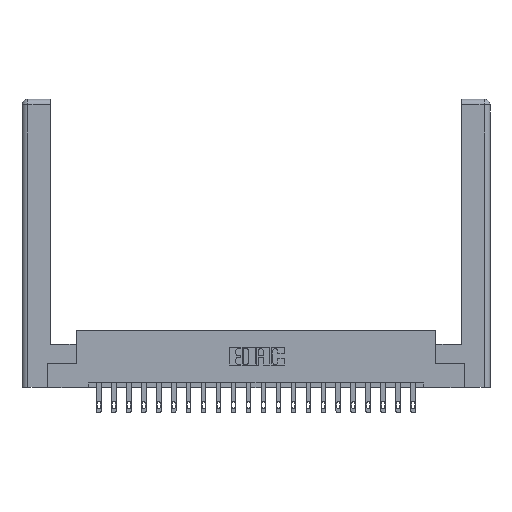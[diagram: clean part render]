
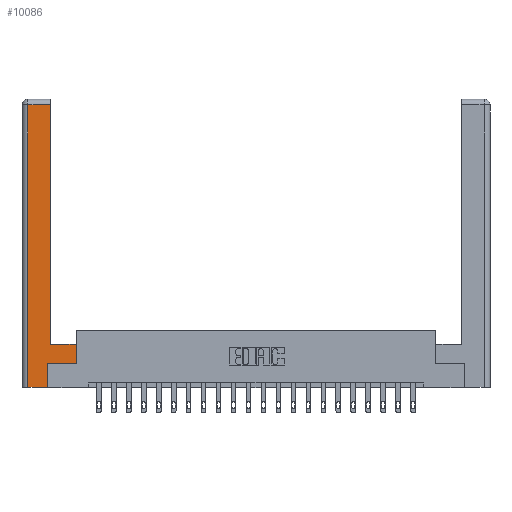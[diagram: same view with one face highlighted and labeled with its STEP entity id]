
A CAD part, top view. The second image highlights one B-rep face of the part: STEP entity #10086.
In plain terms, the highlighted planar face has unit normal (0, 0, 1).
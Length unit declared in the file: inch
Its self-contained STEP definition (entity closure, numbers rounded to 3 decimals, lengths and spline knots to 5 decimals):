
#191 = CARTESIAN_POINT ( 'NONE',  ( 0.565, 0.45, 0. ) ) ;
#448 = CARTESIAN_POINT ( 'NONE',  ( 0.295, 2.94, 0. ) ) ;
#465 = ORIENTED_EDGE ( 'NONE', *, *, #10712, .T. ) ;
#911 = LINE ( 'NONE', #21684, #7870 ) ;
#932 = ORIENTED_EDGE ( 'NONE', *, *, #4241, .T. ) ;
#980 = DIRECTION ( 'NONE',  ( 1., 0., 0. ) ) ;
#1109 = CARTESIAN_POINT ( 'NONE',  ( 0.0615, 2.94, 0. ) ) ;
#1125 = VERTEX_POINT ( 'NONE', #8015 ) ;
#2130 = CARTESIAN_POINT ( 'NONE',  ( 0.295, 0.45, 0. ) ) ;
#2288 = DIRECTION ( 'NONE',  ( -1., 0., 0. ) ) ;
#2538 = ORIENTED_EDGE ( 'NONE', *, *, #7985, .T. ) ;
#2621 = CARTESIAN_POINT ( 'NONE',  ( 0.565, 0.245, 0. ) ) ;
#3746 = VECTOR ( 'NONE', #13568, 39.37008 ) ;
#3827 = CARTESIAN_POINT ( 'NONE',  ( 0.295, 0.45, 0. ) ) ;
#4241 = EDGE_CURVE ( 'NONE', #12772, #1125, #19651, .T. ) ;
#4307 = EDGE_CURVE ( 'NONE', #20152, #16746, #19106, .T. ) ;
#4460 = DIRECTION ( 'NONE',  ( 0., 1., 0. ) ) ;
#4882 = DIRECTION ( 'NONE',  ( 0., -1., 0. ) ) ;
#5393 = VERTEX_POINT ( 'NONE', #7717 ) ;
#5570 = VECTOR ( 'NONE', #4882, 39.37008 ) ;
#6039 = CARTESIAN_POINT ( 'NONE',  ( 0.295, 3., 0. ) ) ;
#6132 = VECTOR ( 'NONE', #18118, 39.37008 ) ;
#6520 = ORIENTED_EDGE ( 'NONE', *, *, #15748, .T. ) ;
#6770 = ORIENTED_EDGE ( 'NONE', *, *, #7977, .T. ) ;
#7197 = LINE ( 'NONE', #9869, #5570 ) ;
#7478 = CARTESIAN_POINT ( 'NONE',  ( 0.0615, 2.94, 0. ) ) ;
#7717 = CARTESIAN_POINT ( 'NONE',  ( 0.565, 0.45, 0. ) ) ;
#7759 = DIRECTION ( 'NONE',  ( -1., 0., 0. ) ) ;
#7870 = VECTOR ( 'NONE', #4460, 39.37008 ) ;
#7977 = EDGE_CURVE ( 'NONE', #16746, #18694, #17577, .T. ) ;
#7985 = EDGE_CURVE ( 'NONE', #11812, #12772, #911, .T. ) ;
#8015 = CARTESIAN_POINT ( 'NONE',  ( 0.565, 0.245, 0. ) ) ;
#8132 = LINE ( 'NONE', #3827, #9222 ) ;
#8241 = EDGE_CURVE ( 'NONE', #5393, #20152, #8132, .T. ) ;
#8368 = EDGE_LOOP ( 'NONE', ( #8949, #6770, #19504, #465, #2538, #932, #6520, #12025 ) ) ;
#8949 = ORIENTED_EDGE ( 'NONE', *, *, #4307, .T. ) ;
#9222 = VECTOR ( 'NONE', #2288, 39.37008 ) ;
#9782 = VECTOR ( 'NONE', #7759, 39.37008 ) ;
#9869 = CARTESIAN_POINT ( 'NONE',  ( 0.0615, 0., 0. ) ) ;
#10086 = ADVANCED_FACE ( 'NONE', ( #16982 ), #16248, .F. ) ;
#10712 = EDGE_CURVE ( 'NONE', #21839, #11812, #14231, .T. ) ;
#11812 = VERTEX_POINT ( 'NONE', #13734 ) ;
#12025 = ORIENTED_EDGE ( 'NONE', *, *, #8241, .T. ) ;
#12772 = VERTEX_POINT ( 'NONE', #15788 ) ;
#13568 = DIRECTION ( 'NONE',  ( 1., 0., 0. ) ) ;
#13734 = CARTESIAN_POINT ( 'NONE',  ( 0.265, 0., 0. ) ) ;
#13785 = CARTESIAN_POINT ( 'NONE',  ( 0.265, 0., 0. ) ) ;
#14231 = LINE ( 'NONE', #13785, #3746 ) ;
#14315 = EDGE_CURVE ( 'NONE', #18694, #21839, #7197, .T. ) ;
#14518 = VECTOR ( 'NONE', #980, 39.37008 ) ;
#14859 = AXIS2_PLACEMENT_3D ( 'NONE', #19494, #21285, #15954 ) ;
#15241 = VECTOR ( 'NONE', #20557, 39.37008 ) ;
#15748 = EDGE_CURVE ( 'NONE', #1125, #5393, #18758, .T. ) ;
#15788 = CARTESIAN_POINT ( 'NONE',  ( 0.265, 0.245, 0. ) ) ;
#15954 = DIRECTION ( 'NONE',  ( -1., 0., 0. ) ) ;
#16248 = PLANE ( 'NONE',  #14859 ) ;
#16746 = VERTEX_POINT ( 'NONE', #448 ) ;
#16982 = FACE_OUTER_BOUND ( 'NONE', #8368, .T. ) ;
#17577 = LINE ( 'NONE', #1109, #9782 ) ;
#18118 = DIRECTION ( 'NONE',  ( 0., 1., 0. ) ) ;
#18694 = VERTEX_POINT ( 'NONE', #7478 ) ;
#18758 = LINE ( 'NONE', #191, #15241 ) ;
#19106 = LINE ( 'NONE', #6039, #6132 ) ;
#19494 = CARTESIAN_POINT ( 'NONE',  ( 0., 0., 0. ) ) ;
#19504 = ORIENTED_EDGE ( 'NONE', *, *, #14315, .T. ) ;
#19651 = LINE ( 'NONE', #2621, #14518 ) ;
#20152 = VERTEX_POINT ( 'NONE', #2130 ) ;
#20557 = DIRECTION ( 'NONE',  ( 0., 1., 0. ) ) ;
#21285 = DIRECTION ( 'NONE',  ( 0., 0., -1. ) ) ;
#21684 = CARTESIAN_POINT ( 'NONE',  ( 0.265, 0.245, 0. ) ) ;
#21832 = CARTESIAN_POINT ( 'NONE',  ( 0.0615, 0., 0. ) ) ;
#21839 = VERTEX_POINT ( 'NONE', #21832 ) ;
